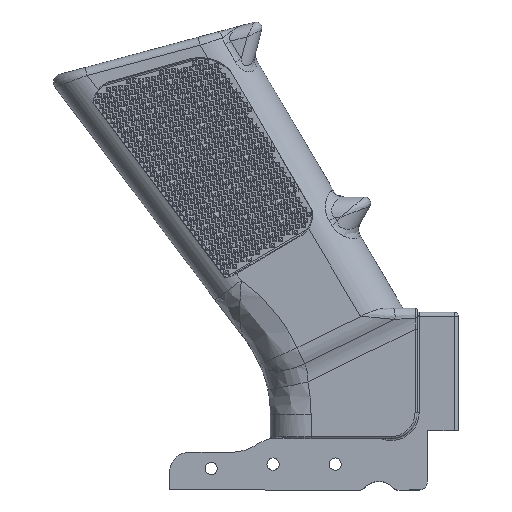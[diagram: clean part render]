
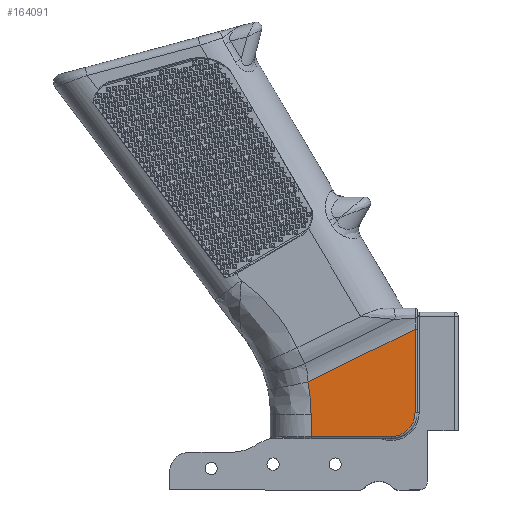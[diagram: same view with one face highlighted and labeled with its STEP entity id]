
A CAD part, front view. The second image highlights one B-rep face of the part: STEP entity #164091.
In plain terms, the highlighted planar face has unit normal (0, -1, 0).
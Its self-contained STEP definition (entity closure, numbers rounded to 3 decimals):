
#3159 = ORIENTED_EDGE ( 'NONE', *, *, #69556, .T. ) ;
#5975 = PLANE ( 'NONE',  #162621 ) ;
#8070 = ORIENTED_EDGE ( 'NONE', *, *, #53556, .T. ) ;
#8440 = CARTESIAN_POINT ( 'NONE',  ( 11.65, 0., -15.5 ) ) ;
#10851 = DIRECTION ( 'NONE',  ( 0., -1., 0. ) ) ;
#15138 = ORIENTED_EDGE ( 'NONE', *, *, #67503, .T. ) ;
#20846 = VERTEX_POINT ( 'NONE', #62550 ) ;
#24236 = DIRECTION ( 'NONE',  ( 0., 0., -1. ) ) ;
#28887 = ORIENTED_EDGE ( 'NONE', *, *, #31468, .T. ) ;
#29920 = EDGE_LOOP ( 'NONE', ( #3159, #28887, #103422, #8070, #98558, #15138 ) ) ;
#30318 = DIRECTION ( 'NONE',  ( 0., -1., 0. ) ) ;
#31099 = VERTEX_POINT ( 'NONE', #136976 ) ;
#31468 = EDGE_CURVE ( 'NONE', #64932, #149076, #81721, .T. ) ;
#36136 = VERTEX_POINT ( 'NONE', #133252 ) ;
#38792 = CARTESIAN_POINT ( 'NONE',  ( -8., 0., 0. ) ) ;
#39141 = CARTESIAN_POINT ( 'NONE',  ( 17.5, 0., 10.789 ) ) ;
#41356 = CARTESIAN_POINT ( 'NONE',  ( -0.861, 0., 1.75 ) ) ;
#42234 = VECTOR ( 'NONE', #129445, 1000. ) ;
#53556 = EDGE_CURVE ( 'NONE', #132708, #36136, #93397, .T. ) ;
#54087 = DIRECTION ( 'NONE',  ( 1., 0., 0. ) ) ;
#56437 = DIRECTION ( 'NONE',  ( -0.897, 0., -0.442 ) ) ;
#56713 = EDGE_CURVE ( 'NONE', #149076, #132708, #155238, .T. ) ;
#58701 = EDGE_CURVE ( 'NONE', #31099, #36136, #83328, .T. ) ;
#60281 = CARTESIAN_POINT ( 'NONE',  ( -8.262, 0., -4.743 ) ) ;
#62550 = CARTESIAN_POINT ( 'NONE',  ( -8., 0., -15.5 ) ) ;
#64932 = VERTEX_POINT ( 'NONE', #8440 ) ;
#66187 = CARTESIAN_POINT ( 'NONE',  ( 17.5, 0., 0. ) ) ;
#67503 = EDGE_CURVE ( 'NONE', #31099, #20846, #153835, .T. ) ;
#69556 = EDGE_CURVE ( 'NONE', #20846, #64932, #143965, .T. ) ;
#79847 = FACE_OUTER_BOUND ( 'NONE', #29920, .T. ) ;
#81721 = CIRCLE ( 'NONE', #143342, 5.85 ) ;
#83328 =( BOUNDED_CURVE ( )  B_SPLINE_CURVE ( 3, ( #125776, #148495, #60281, #162777 ),
 .UNSPECIFIED., .F., .F. ) 
 B_SPLINE_CURVE_WITH_KNOTS ( ( 4, 4 ),
 ( 0., 1. ),
 .UNSPECIFIED. ) 
 CURVE ( )  GEOMETRIC_REPRESENTATION_ITEM ( )  RATIONAL_B_SPLINE_CURVE ( ( 1., 0.997, 0.997, 1. ) ) 
 REPRESENTATION_ITEM ( '' )  );
#86757 = VECTOR ( 'NONE', #143464, 1000. ) ;
#93397 = LINE ( 'NONE', #41356, #127295 ) ;
#98558 = ORIENTED_EDGE ( 'NONE', *, *, #58701, .F. ) ;
#103422 = ORIENTED_EDGE ( 'NONE', *, *, #56713, .T. ) ;
#125776 = CARTESIAN_POINT ( 'NONE',  ( -8., 0., -10.021 ) ) ;
#127295 = VECTOR ( 'NONE', #56437, 1000. ) ;
#129445 = DIRECTION ( 'NONE',  ( 0., 0., -1. ) ) ;
#131337 = CARTESIAN_POINT ( 'NONE',  ( 0., 0., -15.5 ) ) ;
#132708 = VERTEX_POINT ( 'NONE', #39141 ) ;
#132729 = DIRECTION ( 'NONE',  ( 0., 0., -1. ) ) ;
#133252 = CARTESIAN_POINT ( 'NONE',  ( -8.782, 0., -2.15 ) ) ;
#136976 = CARTESIAN_POINT ( 'NONE',  ( -8., 0., -10.021 ) ) ;
#143342 = AXIS2_PLACEMENT_3D ( 'NONE', #161993, #10851, #24236 ) ;
#143464 = DIRECTION ( 'NONE',  ( 0., 0., 1. ) ) ;
#143965 = LINE ( 'NONE', #131337, #155360 ) ;
#145346 = CARTESIAN_POINT ( 'NONE',  ( 0., 0., 0. ) ) ;
#148495 = CARTESIAN_POINT ( 'NONE',  ( -8., 0., -7.376 ) ) ;
#149076 = VERTEX_POINT ( 'NONE', #159487 ) ;
#153835 = LINE ( 'NONE', #38792, #42234 ) ;
#155238 = LINE ( 'NONE', #66187, #86757 ) ;
#155360 = VECTOR ( 'NONE', #54087, 1000. ) ;
#159487 = CARTESIAN_POINT ( 'NONE',  ( 17.5, 0., -9.65 ) ) ;
#161993 = CARTESIAN_POINT ( 'NONE',  ( 11.65, 0., -9.65 ) ) ;
#162621 = AXIS2_PLACEMENT_3D ( 'NONE', #145346, #30318, #132729 ) ;
#162777 = CARTESIAN_POINT ( 'NONE',  ( -8.782, 0., -2.15 ) ) ;
#164091 = ADVANCED_FACE ( 'NONE', ( #79847 ), #5975, .T. ) ;
